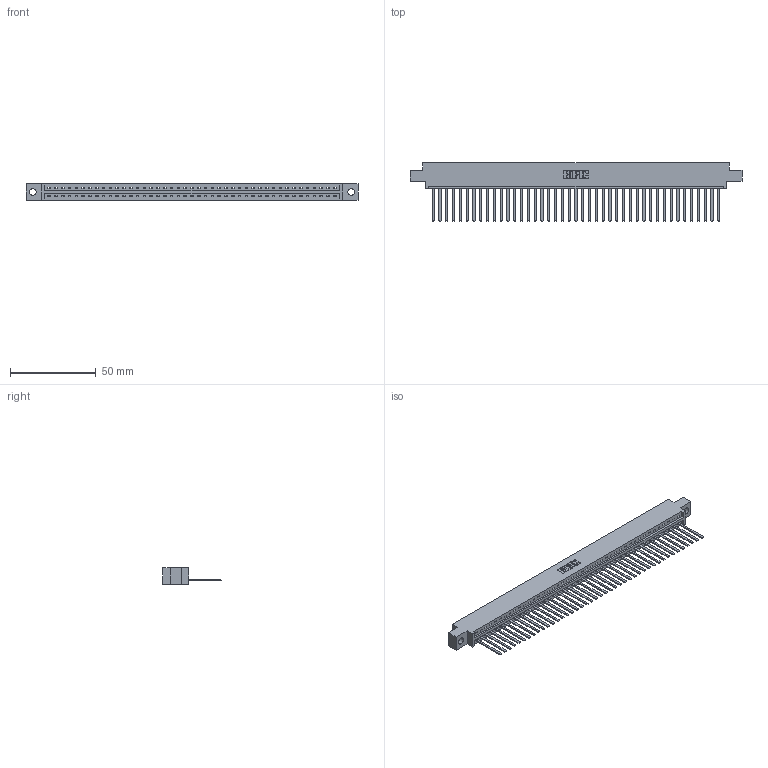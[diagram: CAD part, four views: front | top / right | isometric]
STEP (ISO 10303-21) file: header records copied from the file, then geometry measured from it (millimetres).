
FILE_DESCRIPTION (( 'STEP AP203' ), '1' );
FILE_NAME ('337-043-544-604.STEP', '2018-08-09T03:45:47', ( '' ), ( '' ), 'SwSTEP 2.0', 'SolidWorks 2016', '' );
FILE_SCHEMA (( 'CONFIG_CONTROL_DESIGN' ));
Length unit declared in the file: inch
Products named in the file (3): 337 Part_0.170 Offset - 0.156 Dia-TH; 345-292-001_345-293-144; 337-043-544-604
Assembly tree (44 placements, depth 2):
  337-043-544-604
    337 Part_0.170 Offset - 0.156 Dia-TH
    345-292-001_345-293-144  x43
Bounding box: 193.4 x 34.3 x 9.4 mm (x, y, z)
Volume: 20405.4 mm3; surface area: 22621.4 mm2
Topology: 44 solids, 44 shells, 2526 faces, 7633 edges, 5030 vertices
Faces by surface type: plane 1880, cylinder 646
Entity records: 31785 total; most frequent: CARTESIAN_POINT 5543, ORIENTED_EDGE 5522, DIRECTION 4659, EDGE_CURVE 2761, VECTOR 2637, LINE 2637, VERTEX_POINT 1838, AXIS2_PLACEMENT_3D 1011
